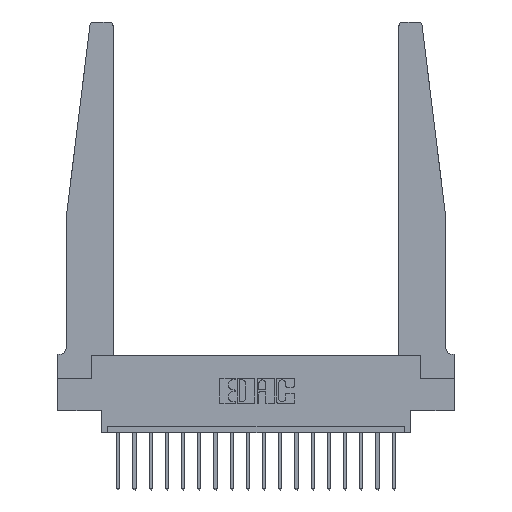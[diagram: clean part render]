
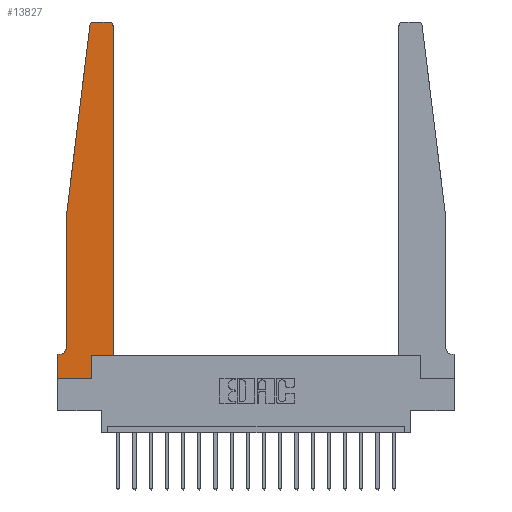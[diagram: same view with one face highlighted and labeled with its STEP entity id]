
A CAD part, top view. The second image highlights one B-rep face of the part: STEP entity #13827.
In plain terms, the highlighted planar face has unit normal (0, 0, 1).
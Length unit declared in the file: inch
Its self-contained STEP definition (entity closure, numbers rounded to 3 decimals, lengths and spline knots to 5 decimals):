
#134 = ORIENTED_EDGE ( 'NONE', *, *, #3836, .T. ) ;
#186 = CARTESIAN_POINT ( 'NONE',  ( 0.2605, 0.18, 0.37 ) ) ;
#378 = CARTESIAN_POINT ( 'NONE',  ( 0.2605, 0., 0.37 ) ) ;
#392 = DIRECTION ( 'NONE',  ( 1., 0., 0. ) ) ;
#499 = DIRECTION ( 'NONE',  ( 0., 0., 1. ) ) ;
#884 = EDGE_LOOP ( 'NONE', ( #10083, #7880, #2400, #5831, #6832, #2156, #4948, #134, #10305, #14030, #3589, #1945 ) ) ;
#1008 = CARTESIAN_POINT ( 'NONE',  ( 0.395, 2.75, 0.37 ) ) ;
#1044 = CIRCLE ( 'NONE', #1365, 0.05 ) ;
#1084 = LINE ( 'NONE', #6999, #17650 ) ;
#1337 = EDGE_CURVE ( 'NONE', #16868, #2124, #11064, .T. ) ;
#1365 = AXIS2_PLACEMENT_3D ( 'NONE', #12764, #8359, #14448 ) ;
#1384 = EDGE_CURVE ( 'NONE', #3768, #2781, #1657, .T. ) ;
#1657 = LINE ( 'NONE', #11841, #3725 ) ;
#1945 = ORIENTED_EDGE ( 'NONE', *, *, #14841, .T. ) ;
#1969 = CARTESIAN_POINT ( 'NONE',  ( 0.425, 0.18, 0.37 ) ) ;
#2124 = VERTEX_POINT ( 'NONE', #6610 ) ;
#2156 = ORIENTED_EDGE ( 'NONE', *, *, #11640, .T. ) ;
#2400 = ORIENTED_EDGE ( 'NONE', *, *, #17867, .T. ) ;
#2537 = DIRECTION ( 'NONE',  ( 0., 1., 0. ) ) ;
#2577 = DIRECTION ( 'NONE',  ( 0., 0., 1. ) ) ;
#2781 = VERTEX_POINT ( 'NONE', #5570 ) ;
#2867 = DIRECTION ( 'NONE',  ( 0., 0., 1. ) ) ;
#3497 = LINE ( 'NONE', #15960, #4896 ) ;
#3589 = ORIENTED_EDGE ( 'NONE', *, *, #15797, .T. ) ;
#3725 = VECTOR ( 'NONE', #13442, 39.37008 ) ;
#3768 = VERTEX_POINT ( 'NONE', #11471 ) ;
#3836 = EDGE_CURVE ( 'NONE', #15275, #10515, #3497, .T. ) ;
#4222 = VECTOR ( 'NONE', #8062, 39.37008 ) ;
#4344 = DIRECTION ( 'NONE',  ( -0.122, -0.992, 0. ) ) ;
#4581 = CARTESIAN_POINT ( 'NONE',  ( 0.065, 0.1875, 0.37 ) ) ;
#4679 = AXIS2_PLACEMENT_3D ( 'NONE', #10653, #2867, #18341 ) ;
#4857 = CARTESIAN_POINT ( 'NONE',  ( 0.25, 2.75, 0.37 ) ) ;
#4893 = CARTESIAN_POINT ( 'NONE',  ( 0.395, 2.72, 0.37 ) ) ;
#4896 = VECTOR ( 'NONE', #392, 39.37008 ) ;
#4948 = ORIENTED_EDGE ( 'NONE', *, *, #12477, .T. ) ;
#4957 = DIRECTION ( 'NONE',  ( -1., 0., 0. ) ) ;
#5347 = VECTOR ( 'NONE', #4344, 39.37008 ) ;
#5401 = DIRECTION ( 'NONE',  ( 0., -1., 0. ) ) ;
#5570 = CARTESIAN_POINT ( 'NONE',  ( 0.065, 0.2375, 0.37 ) ) ;
#5648 = CARTESIAN_POINT ( 'NONE',  ( 0.27653, 2.75, 0.37 ) ) ;
#5831 = ORIENTED_EDGE ( 'NONE', *, *, #1384, .T. ) ;
#5945 = CARTESIAN_POINT ( 'NONE',  ( 0.425, 0.18, 0.37 ) ) ;
#6610 = CARTESIAN_POINT ( 'NONE',  ( 0.24675, 2.72367, 0.37 ) ) ;
#6639 = DIRECTION ( 'NONE',  ( 0., 1., 0. ) ) ;
#6774 = FACE_OUTER_BOUND ( 'NONE', #884, .T. ) ;
#6832 = ORIENTED_EDGE ( 'NONE', *, *, #12955, .T. ) ;
#6999 = CARTESIAN_POINT ( 'NONE',  ( 0., 0., 0.37 ) ) ;
#7129 = VECTOR ( 'NONE', #13969, 39.37008 ) ;
#7415 = CARTESIAN_POINT ( 'NONE',  ( 0., 0.1875, 0.37 ) ) ;
#7725 = CARTESIAN_POINT ( 'NONE',  ( 0.015, 0.1875, 0.37 ) ) ;
#7744 = VERTEX_POINT ( 'NONE', #7415 ) ;
#7880 = ORIENTED_EDGE ( 'NONE', *, *, #1337, .T. ) ;
#8062 = DIRECTION ( 'NONE',  ( 1., 0., 0. ) ) ;
#8283 = DIRECTION ( 'NONE',  ( 1., 0., 0. ) ) ;
#8359 = DIRECTION ( 'NONE',  ( 0., 0., -1. ) ) ;
#8504 = VERTEX_POINT ( 'NONE', #5945 ) ;
#8511 = CIRCLE ( 'NONE', #17130, 0.03 ) ;
#9234 = VERTEX_POINT ( 'NONE', #11981 ) ;
#10083 = ORIENTED_EDGE ( 'NONE', *, *, #17702, .T. ) ;
#10305 = ORIENTED_EDGE ( 'NONE', *, *, #14134, .T. ) ;
#10515 = VERTEX_POINT ( 'NONE', #378 ) ;
#10615 = EDGE_CURVE ( 'NONE', #9234, #8504, #15746, .T. ) ;
#10653 = CARTESIAN_POINT ( 'NONE',  ( 0.27653, 2.72, 0.37 ) ) ;
#10785 = LINE ( 'NONE', #4581, #7129 ) ;
#10959 = CARTESIAN_POINT ( 'NONE',  ( 0., 0., 0.37 ) ) ;
#11037 = VECTOR ( 'NONE', #6639, 39.37008 ) ;
#11064 = CIRCLE ( 'NONE', #4679, 0.03 ) ;
#11471 = CARTESIAN_POINT ( 'NONE',  ( 0.065, 1.25, 0.37 ) ) ;
#11640 = EDGE_CURVE ( 'NONE', #13573, #7744, #10785, .T. ) ;
#11665 = CARTESIAN_POINT ( 'NONE',  ( 0., 0.1875, 0.37 ) ) ;
#11727 = VECTOR ( 'NONE', #4957, 39.37008 ) ;
#11841 = CARTESIAN_POINT ( 'NONE',  ( 0.065, 1.25, 0.37 ) ) ;
#11981 = CARTESIAN_POINT ( 'NONE',  ( 0.2605, 0.18, 0.37 ) ) ;
#12028 = LINE ( 'NONE', #17824, #5347 ) ;
#12477 = EDGE_CURVE ( 'NONE', #7744, #15275, #1084, .T. ) ;
#12629 = AXIS2_PLACEMENT_3D ( 'NONE', #11665, #2577, #16061 ) ;
#12764 = CARTESIAN_POINT ( 'NONE',  ( 0.015, 0.2375, 0.37 ) ) ;
#12824 = CARTESIAN_POINT ( 'NONE',  ( 0.425, 0.18, 0.37 ) ) ;
#12887 = CARTESIAN_POINT ( 'NONE',  ( 0.425, 2.72, 0.37 ) ) ;
#12955 = EDGE_CURVE ( 'NONE', #2781, #13573, #1044, .T. ) ;
#13442 = DIRECTION ( 'NONE',  ( 0., -1., 0. ) ) ;
#13573 = VERTEX_POINT ( 'NONE', #7725 ) ;
#13827 = ADVANCED_FACE ( 'NONE', ( #6774 ), #17363, .T. ) ;
#13969 = DIRECTION ( 'NONE',  ( -1., 0., 0. ) ) ;
#14030 = ORIENTED_EDGE ( 'NONE', *, *, #10615, .T. ) ;
#14134 = EDGE_CURVE ( 'NONE', #10515, #9234, #16869, .T. ) ;
#14448 = DIRECTION ( 'NONE',  ( -1., 0., 0. ) ) ;
#14657 = VERTEX_POINT ( 'NONE', #1008 ) ;
#14841 = EDGE_CURVE ( 'NONE', #19558, #14657, #8511, .T. ) ;
#15275 = VERTEX_POINT ( 'NONE', #10959 ) ;
#15746 = LINE ( 'NONE', #1969, #4222 ) ;
#15797 = EDGE_CURVE ( 'NONE', #8504, #19558, #16020, .T. ) ;
#15960 = CARTESIAN_POINT ( 'NONE',  ( 0., 0., 0.37 ) ) ;
#16020 = LINE ( 'NONE', #12824, #18040 ) ;
#16061 = DIRECTION ( 'NONE',  ( 1., 0., 0. ) ) ;
#16868 = VERTEX_POINT ( 'NONE', #5648 ) ;
#16869 = LINE ( 'NONE', #186, #11037 ) ;
#17130 = AXIS2_PLACEMENT_3D ( 'NONE', #4893, #499, #8283 ) ;
#17363 = PLANE ( 'NONE',  #12629 ) ;
#17650 = VECTOR ( 'NONE', #5401, 39.37008 ) ;
#17702 = EDGE_CURVE ( 'NONE', #14657, #16868, #18536, .T. ) ;
#17824 = CARTESIAN_POINT ( 'NONE',  ( 0.065, 1.25, 0.37 ) ) ;
#17867 = EDGE_CURVE ( 'NONE', #2124, #3768, #12028, .T. ) ;
#18040 = VECTOR ( 'NONE', #2537, 39.37008 ) ;
#18341 = DIRECTION ( 'NONE',  ( 1., 0., 0. ) ) ;
#18536 = LINE ( 'NONE', #4857, #11727 ) ;
#19558 = VERTEX_POINT ( 'NONE', #12887 ) ;
